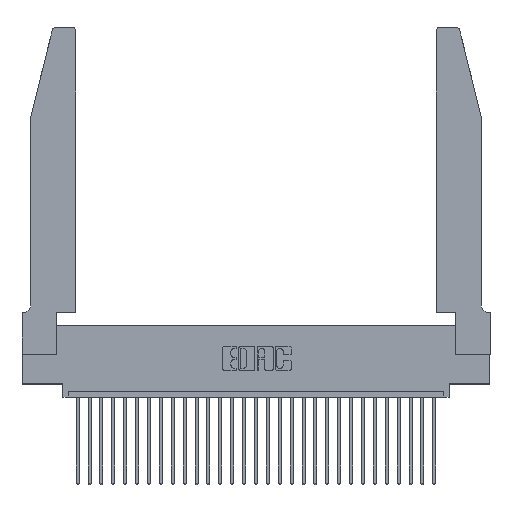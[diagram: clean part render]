
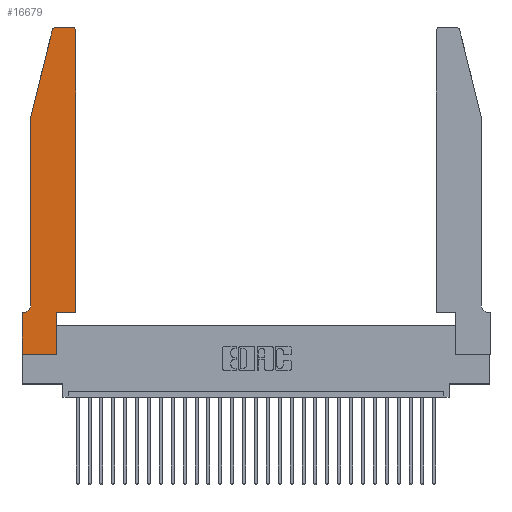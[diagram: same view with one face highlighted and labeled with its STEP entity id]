
A CAD part, top view. The second image highlights one B-rep face of the part: STEP entity #16679.
In plain terms, the highlighted planar face has unit normal (0, 0, 1).
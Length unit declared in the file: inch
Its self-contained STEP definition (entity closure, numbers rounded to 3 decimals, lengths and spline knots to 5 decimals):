
#535 = CARTESIAN_POINT ( 'NONE',  ( 0.0755, 2., 0.37 ) ) ;
#1071 = DIRECTION ( 'NONE',  ( 1., 0., 0. ) ) ;
#1118 = CARTESIAN_POINT ( 'NONE',  ( 0.0055, 0.35, 0.37 ) ) ;
#1191 = VERTEX_POINT ( 'NONE', #11125 ) ;
#1285 = DIRECTION ( 'NONE',  ( 1., 0., 0. ) ) ;
#1366 = CARTESIAN_POINT ( 'NONE',  ( 0.284, 2.75, 0.37 ) ) ;
#1868 = VERTEX_POINT ( 'NONE', #3870 ) ;
#2162 = EDGE_CURVE ( 'NONE', #1868, #1191, #3611, .T. ) ;
#2643 = ORIENTED_EDGE ( 'NONE', *, *, #16804, .T. ) ;
#2798 = VERTEX_POINT ( 'NONE', #23939 ) ;
#3254 = CIRCLE ( 'NONE', #3679, 0.07 ) ;
#3611 = LINE ( 'NONE', #20970, #8960 ) ;
#3630 = LINE ( 'NONE', #9213, #29112 ) ;
#3679 = AXIS2_PLACEMENT_3D ( 'NONE', #18343, #25181, #28134 ) ;
#3870 = CARTESIAN_POINT ( 'NONE',  ( 0.4505, 0.35, 0.37 ) ) ;
#4538 = VECTOR ( 'NONE', #18847, 39.37008 ) ;
#4738 = DIRECTION ( 'NONE',  ( -1., 0., 0. ) ) ;
#5078 = DIRECTION ( 'NONE',  ( 0., -1., 0. ) ) ;
#5784 = ORIENTED_EDGE ( 'NONE', *, *, #17936, .T. ) ;
#6318 = CARTESIAN_POINT ( 'NONE',  ( 0.2865, 0., 0.37 ) ) ;
#7266 = DIRECTION ( 'NONE',  ( 0., 1., 0. ) ) ;
#7422 = CIRCLE ( 'NONE', #25208, 0.03 ) ;
#7512 = CARTESIAN_POINT ( 'NONE',  ( 0.284, 2.72, 0.37 ) ) ;
#7919 = DIRECTION ( 'NONE',  ( 0., 0., 1. ) ) ;
#8405 = ORIENTED_EDGE ( 'NONE', *, *, #19398, .T. ) ;
#8408 = CARTESIAN_POINT ( 'NONE',  ( 0.0755, 2., 0.37 ) ) ;
#8497 = VECTOR ( 'NONE', #1071, 39.37008 ) ;
#8587 = VERTEX_POINT ( 'NONE', #8408 ) ;
#8668 = VERTEX_POINT ( 'NONE', #24525 ) ;
#8780 = LINE ( 'NONE', #27310, #24287 ) ;
#8960 = VECTOR ( 'NONE', #7266, 39.37008 ) ;
#9213 = CARTESIAN_POINT ( 'NONE',  ( 0.0755, 0.35, 0.37 ) ) ;
#10264 = LINE ( 'NONE', #14772, #8497 ) ;
#10331 = VERTEX_POINT ( 'NONE', #28121 ) ;
#10549 = PLANE ( 'NONE',  #19384 ) ;
#10554 = ORIENTED_EDGE ( 'NONE', *, *, #25611, .T. ) ;
#10994 = LINE ( 'NONE', #535, #16681 ) ;
#11125 = CARTESIAN_POINT ( 'NONE',  ( 0.4505, 2.72, 0.37 ) ) ;
#13843 = LINE ( 'NONE', #15408, #4538 ) ;
#13953 = DIRECTION ( 'NONE',  ( 0., 1., 0. ) ) ;
#14055 = VERTEX_POINT ( 'NONE', #17880 ) ;
#14277 = FACE_OUTER_BOUND ( 'NONE', #18895, .T. ) ;
#14665 = ORIENTED_EDGE ( 'NONE', *, *, #20725, .T. ) ;
#14772 = CARTESIAN_POINT ( 'NONE',  ( 0.4505, 0.35, 0.37 ) ) ;
#14837 = ORIENTED_EDGE ( 'NONE', *, *, #18264, .T. ) ;
#14991 = LINE ( 'NONE', #20469, #15698 ) ;
#14994 = LINE ( 'NONE', #16493, #26198 ) ;
#15408 = CARTESIAN_POINT ( 'NONE',  ( 0., 0., 0.37 ) ) ;
#15698 = VECTOR ( 'NONE', #13953, 39.37008 ) ;
#16493 = CARTESIAN_POINT ( 'NONE',  ( 0., 0., 0.37 ) ) ;
#16679 = ADVANCED_FACE ( 'NONE', ( #14277 ), #10549, .T. ) ;
#16681 = VECTOR ( 'NONE', #18845, 39.37008 ) ;
#16804 = EDGE_CURVE ( 'NONE', #28178, #8668, #14991, .T. ) ;
#16819 = EDGE_CURVE ( 'NONE', #1191, #10331, #7422, .T. ) ;
#16857 = DIRECTION ( 'NONE',  ( 1., 0., 0. ) ) ;
#17880 = CARTESIAN_POINT ( 'NONE',  ( 0., 0., 0.37 ) ) ;
#17936 = EDGE_CURVE ( 'NONE', #8668, #1868, #10264, .T. ) ;
#18264 = EDGE_CURVE ( 'NONE', #14055, #28178, #13843, .T. ) ;
#18343 = CARTESIAN_POINT ( 'NONE',  ( 0.0055, 0.42, 0.37 ) ) ;
#18478 = VERTEX_POINT ( 'NONE', #21576 ) ;
#18845 = DIRECTION ( 'NONE',  ( 0., -1., 0. ) ) ;
#18847 = DIRECTION ( 'NONE',  ( 1., 0., 0. ) ) ;
#18895 = EDGE_LOOP ( 'NONE', ( #8405, #14665, #22990, #21509, #10554, #23312, #20692, #14837, #2643, #5784, #28459, #28834 ) ) ;
#18988 = EDGE_CURVE ( 'NONE', #18478, #8587, #23975, .T. ) ;
#19214 = DIRECTION ( 'NONE',  ( -0.239, -0.971, 0. ) ) ;
#19384 = AXIS2_PLACEMENT_3D ( 'NONE', #28865, #19733, #1285 ) ;
#19398 = EDGE_CURVE ( 'NONE', #10331, #21445, #8780, .T. ) ;
#19733 = DIRECTION ( 'NONE',  ( 0., 0., 1. ) ) ;
#20346 = VERTEX_POINT ( 'NONE', #23500 ) ;
#20458 = EDGE_CURVE ( 'NONE', #20346, #14055, #14994, .T. ) ;
#20469 = CARTESIAN_POINT ( 'NONE',  ( 0.2865, 0.35, 0.37 ) ) ;
#20692 = ORIENTED_EDGE ( 'NONE', *, *, #20458, .T. ) ;
#20725 = EDGE_CURVE ( 'NONE', #21445, #18478, #26085, .T. ) ;
#20970 = CARTESIAN_POINT ( 'NONE',  ( 0.4505, 0.35, 0.37 ) ) ;
#21225 = EDGE_CURVE ( 'NONE', #8587, #2798, #10994, .T. ) ;
#21445 = VERTEX_POINT ( 'NONE', #1366 ) ;
#21509 = ORIENTED_EDGE ( 'NONE', *, *, #21225, .T. ) ;
#21576 = CARTESIAN_POINT ( 'NONE',  ( 0.25487, 2.72718, 0.37 ) ) ;
#22548 = AXIS2_PLACEMENT_3D ( 'NONE', #7512, #7919, #28431 ) ;
#22990 = ORIENTED_EDGE ( 'NONE', *, *, #18988, .T. ) ;
#23312 = ORIENTED_EDGE ( 'NONE', *, *, #25615, .T. ) ;
#23500 = CARTESIAN_POINT ( 'NONE',  ( 0., 0.35, 0.37 ) ) ;
#23939 = CARTESIAN_POINT ( 'NONE',  ( 0.0755, 0.42, 0.37 ) ) ;
#23975 = LINE ( 'NONE', #28171, #29319 ) ;
#24287 = VECTOR ( 'NONE', #4738, 39.37008 ) ;
#24525 = CARTESIAN_POINT ( 'NONE',  ( 0.2865, 0.35, 0.37 ) ) ;
#24750 = VERTEX_POINT ( 'NONE', #1118 ) ;
#25181 = DIRECTION ( 'NONE',  ( 0., 0., -1. ) ) ;
#25208 = AXIS2_PLACEMENT_3D ( 'NONE', #25887, #28557, #16857 ) ;
#25611 = EDGE_CURVE ( 'NONE', #2798, #24750, #3254, .T. ) ;
#25615 = EDGE_CURVE ( 'NONE', #24750, #20346, #3630, .T. ) ;
#25887 = CARTESIAN_POINT ( 'NONE',  ( 0.4205, 2.72, 0.37 ) ) ;
#26085 = CIRCLE ( 'NONE', #22548, 0.03 ) ;
#26198 = VECTOR ( 'NONE', #5078, 39.37008 ) ;
#27310 = CARTESIAN_POINT ( 'NONE',  ( 0.2605, 2.75, 0.37 ) ) ;
#27388 = DIRECTION ( 'NONE',  ( -1., 0., 0. ) ) ;
#28121 = CARTESIAN_POINT ( 'NONE',  ( 0.4205, 2.75, 0.37 ) ) ;
#28134 = DIRECTION ( 'NONE',  ( -1., 0., 0. ) ) ;
#28171 = CARTESIAN_POINT ( 'NONE',  ( 0.0755, 2., 0.37 ) ) ;
#28178 = VERTEX_POINT ( 'NONE', #6318 ) ;
#28431 = DIRECTION ( 'NONE',  ( 1., 0., 0. ) ) ;
#28459 = ORIENTED_EDGE ( 'NONE', *, *, #2162, .T. ) ;
#28557 = DIRECTION ( 'NONE',  ( 0., 0., 1. ) ) ;
#28834 = ORIENTED_EDGE ( 'NONE', *, *, #16819, .T. ) ;
#28865 = CARTESIAN_POINT ( 'NONE',  ( 0., 0.35, 0.37 ) ) ;
#29112 = VECTOR ( 'NONE', #27388, 39.37008 ) ;
#29319 = VECTOR ( 'NONE', #19214, 39.37008 ) ;
